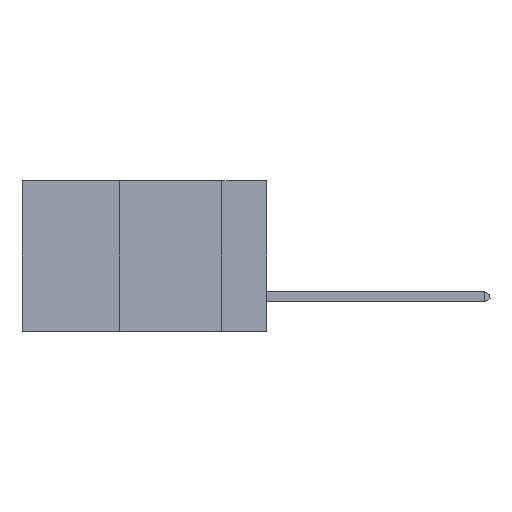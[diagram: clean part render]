
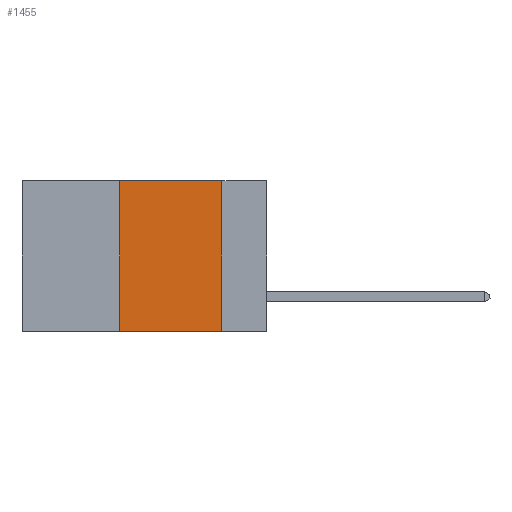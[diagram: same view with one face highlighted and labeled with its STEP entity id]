
A CAD part, left-side view. The second image highlights one B-rep face of the part: STEP entity #1455.
In plain terms, the highlighted planar face has unit normal (-1, 0, 0).
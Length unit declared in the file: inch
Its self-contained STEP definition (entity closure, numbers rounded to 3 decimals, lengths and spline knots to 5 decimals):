
#240 = DIRECTION ( 'NONE',  ( 1., 0., 0. ) ) ;
#567 = FACE_OUTER_BOUND ( 'NONE', #9112, .T. ) ;
#648 = VECTOR ( 'NONE', #9202, 39.37008 ) ;
#1206 = LINE ( 'NONE', #13380, #7358 ) ;
#1207 = DIRECTION ( 'NONE',  ( 0., -1., 0. ) ) ;
#1400 = PLANE ( 'NONE',  #8243 ) ;
#1444 = VERTEX_POINT ( 'NONE', #3638 ) ;
#1455 = ADVANCED_FACE ( 'NONE', ( #567 ), #1400, .F. ) ;
#1550 = ORIENTED_EDGE ( 'NONE', *, *, #7166, .F. ) ;
#1788 = ORIENTED_EDGE ( 'NONE', *, *, #10836, .F. ) ;
#1933 = VERTEX_POINT ( 'NONE', #7066 ) ;
#2151 = ORIENTED_EDGE ( 'NONE', *, *, #9210, .F. ) ;
#2215 = ORIENTED_EDGE ( 'NONE', *, *, #6609, .T. ) ;
#3282 = VERTEX_POINT ( 'NONE', #11450 ) ;
#3638 = CARTESIAN_POINT ( 'NONE',  ( 0., 0.36, -0.37 ) ) ;
#4037 = LINE ( 'NONE', #8045, #648 ) ;
#4637 = DIRECTION ( 'NONE',  ( 0., 0., -1. ) ) ;
#5024 = CARTESIAN_POINT ( 'NONE',  ( 0., 0.6, -0.37 ) ) ;
#6274 = CARTESIAN_POINT ( 'NONE',  ( 0., 0.6, 0. ) ) ;
#6609 = EDGE_CURVE ( 'NONE', #1444, #13503, #7031, .T. ) ;
#6702 = VECTOR ( 'NONE', #10612, 39.37008 ) ;
#7031 = LINE ( 'NONE', #5024, #6702 ) ;
#7066 = CARTESIAN_POINT ( 'NONE',  ( 0., 0.11, 0. ) ) ;
#7127 = CARTESIAN_POINT ( 'NONE',  ( 0., 0.6, 0. ) ) ;
#7166 = EDGE_CURVE ( 'NONE', #1933, #13503, #4037, .T. ) ;
#7358 = VECTOR ( 'NONE', #14282, 39.37008 ) ;
#8045 = CARTESIAN_POINT ( 'NONE',  ( 0., 0.11, 0. ) ) ;
#8243 = AXIS2_PLACEMENT_3D ( 'NONE', #7127, #240, #4637 ) ;
#9112 = EDGE_LOOP ( 'NONE', ( #1550, #1788, #2151, #2215 ) ) ;
#9202 = DIRECTION ( 'NONE',  ( 0., 0., -1. ) ) ;
#9210 = EDGE_CURVE ( 'NONE', #1444, #3282, #1206, .T. ) ;
#10612 = DIRECTION ( 'NONE',  ( 0., -1., 0. ) ) ;
#10836 = EDGE_CURVE ( 'NONE', #3282, #1933, #12059, .T. ) ;
#11450 = CARTESIAN_POINT ( 'NONE',  ( 0., 0.36, 0. ) ) ;
#11591 = CARTESIAN_POINT ( 'NONE',  ( 0., 0.11, -0.37 ) ) ;
#11726 = VECTOR ( 'NONE', #1207, 39.37008 ) ;
#12059 = LINE ( 'NONE', #6274, #11726 ) ;
#13380 = CARTESIAN_POINT ( 'NONE',  ( 0., 0.36, 0. ) ) ;
#13503 = VERTEX_POINT ( 'NONE', #11591 ) ;
#14282 = DIRECTION ( 'NONE',  ( 0., 0., 1. ) ) ;
